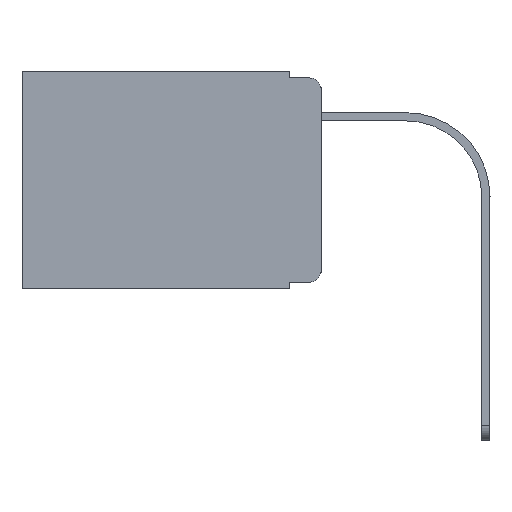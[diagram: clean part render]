
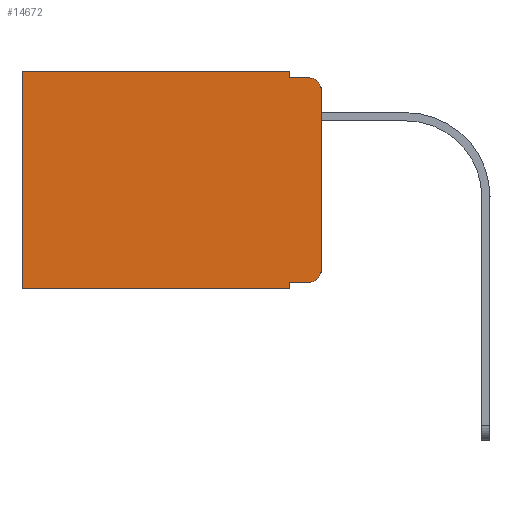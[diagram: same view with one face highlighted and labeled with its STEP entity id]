
A CAD part, left-side view. The second image highlights one B-rep face of the part: STEP entity #14672.
In plain terms, the highlighted planar face has unit normal (-1, 0, 0).
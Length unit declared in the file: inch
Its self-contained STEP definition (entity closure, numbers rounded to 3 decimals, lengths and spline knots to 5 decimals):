
#27 = VERTEX_POINT ( 'NONE', #1675 ) ;
#57 = CARTESIAN_POINT ( 'NONE',  ( 0.298, 0.02, -0.03 ) ) ;
#279 = CARTESIAN_POINT ( 'NONE',  ( 0.298, 0.051, 0. ) ) ;
#735 = ORIENTED_EDGE ( 'NONE', *, *, #15485, .T. ) ;
#769 = VERTEX_POINT ( 'NONE', #1514 ) ;
#1252 = VERTEX_POINT ( 'NONE', #11580 ) ;
#1514 = CARTESIAN_POINT ( 'NONE',  ( 0.298, 0.051, -0.01 ) ) ;
#1627 = PLANE ( 'NONE',  #4900 ) ;
#1675 = CARTESIAN_POINT ( 'NONE',  ( 0.298, 0.051, 0. ) ) ;
#1926 = ORIENTED_EDGE ( 'NONE', *, *, #7723, .T. ) ;
#2039 = EDGE_CURVE ( 'NONE', #3772, #8270, #19873, .T. ) ;
#2563 = VERTEX_POINT ( 'NONE', #8257 ) ;
#2780 = CARTESIAN_POINT ( 'NONE',  ( 0.298, 0.02, -0.01 ) ) ;
#3042 = CIRCLE ( 'NONE', #18244, 0.02 ) ;
#3081 = DIRECTION ( 'NONE',  ( 0., 0., -1. ) ) ;
#3502 = DIRECTION ( 'NONE',  ( 0., 0., -1. ) ) ;
#3566 = LINE ( 'NONE', #17082, #7399 ) ;
#3606 = ORIENTED_EDGE ( 'NONE', *, *, #2039, .T. ) ;
#3688 = LINE ( 'NONE', #20299, #4936 ) ;
#3772 = VERTEX_POINT ( 'NONE', #16902 ) ;
#3963 = LINE ( 'NONE', #7512, #16135 ) ;
#4053 = LINE ( 'NONE', #7702, #10940 ) ;
#4299 = CARTESIAN_POINT ( 'NONE',  ( 0.298, 0.473, 0. ) ) ;
#4418 = DIRECTION ( 'NONE',  ( 0., 0., -1. ) ) ;
#4834 = CARTESIAN_POINT ( 'NONE',  ( 0.298, 0.051, -0.01 ) ) ;
#4900 = AXIS2_PLACEMENT_3D ( 'NONE', #15141, #15360, #3081 ) ;
#4936 = VECTOR ( 'NONE', #20626, 39.37008 ) ;
#5327 = ORIENTED_EDGE ( 'NONE', *, *, #12393, .F. ) ;
#5616 = VECTOR ( 'NONE', #6398, 39.37008 ) ;
#6398 = DIRECTION ( 'NONE',  ( 0., -1., 0. ) ) ;
#6643 = ORIENTED_EDGE ( 'NONE', *, *, #14414, .F. ) ;
#7184 = VERTEX_POINT ( 'NONE', #17137 ) ;
#7365 = EDGE_CURVE ( 'NONE', #27, #10118, #3963, .T. ) ;
#7399 = VECTOR ( 'NONE', #19055, 39.37008 ) ;
#7512 = CARTESIAN_POINT ( 'NONE',  ( 0.298, 0., 0. ) ) ;
#7702 = CARTESIAN_POINT ( 'NONE',  ( 0.298, 0., 0. ) ) ;
#7723 = EDGE_CURVE ( 'NONE', #1252, #19000, #3042, .T. ) ;
#8257 = CARTESIAN_POINT ( 'NONE',  ( 0.298, 0.051, -0.333 ) ) ;
#8270 = VERTEX_POINT ( 'NONE', #9193 ) ;
#8373 = CARTESIAN_POINT ( 'NONE',  ( 0.298, 0.473, 0. ) ) ;
#9161 = DIRECTION ( 'NONE',  ( 0., 1., 0. ) ) ;
#9193 = CARTESIAN_POINT ( 'NONE',  ( 0.298, 0., -0.313 ) ) ;
#9301 = ORIENTED_EDGE ( 'NONE', *, *, #10661, .F. ) ;
#9907 = EDGE_CURVE ( 'NONE', #2563, #3772, #12373, .T. ) ;
#10118 = VERTEX_POINT ( 'NONE', #8373 ) ;
#10119 = EDGE_CURVE ( 'NONE', #769, #19000, #19993, .T. ) ;
#10338 = AXIS2_PLACEMENT_3D ( 'NONE', #13040, #18247, #4418 ) ;
#10351 = EDGE_CURVE ( 'NONE', #1252, #8270, #4053, .T. ) ;
#10617 = CARTESIAN_POINT ( 'NONE',  ( 0.298, 0.051, -0.333 ) ) ;
#10661 = EDGE_CURVE ( 'NONE', #18997, #7184, #3688, .T. ) ;
#10940 = VECTOR ( 'NONE', #16014, 39.37008 ) ;
#11580 = CARTESIAN_POINT ( 'NONE',  ( 0.298, 0., -0.03 ) ) ;
#12355 = VECTOR ( 'NONE', #3502, 39.37008 ) ;
#12373 = LINE ( 'NONE', #10617, #17623 ) ;
#12393 = EDGE_CURVE ( 'NONE', #27, #769, #15458, .T. ) ;
#13040 = CARTESIAN_POINT ( 'NONE',  ( 0.298, 0.02, -0.313 ) ) ;
#13249 = FACE_OUTER_BOUND ( 'NONE', #14753, .T. ) ;
#13452 = DIRECTION ( 'NONE',  ( -1., 0., 0. ) ) ;
#13640 = ORIENTED_EDGE ( 'NONE', *, *, #10119, .F. ) ;
#13667 = DIRECTION ( 'NONE',  ( 0., 0., -1. ) ) ;
#14414 = EDGE_CURVE ( 'NONE', #2563, #18997, #3566, .T. ) ;
#14672 = ADVANCED_FACE ( 'NONE', ( #13249 ), #1627, .F. ) ;
#14753 = EDGE_LOOP ( 'NONE', ( #19637, #1926, #13640, #5327, #19267, #735, #9301, #6643, #16917, #3606 ) ) ;
#14939 = VECTOR ( 'NONE', #19568, 39.37008 ) ;
#15141 = CARTESIAN_POINT ( 'NONE',  ( 0.298, 0., 0. ) ) ;
#15360 = DIRECTION ( 'NONE',  ( 1., 0., 0. ) ) ;
#15458 = LINE ( 'NONE', #279, #12355 ) ;
#15485 = EDGE_CURVE ( 'NONE', #10118, #7184, #16141, .T. ) ;
#16014 = DIRECTION ( 'NONE',  ( 0., 0., -1. ) ) ;
#16135 = VECTOR ( 'NONE', #9161, 39.37008 ) ;
#16141 = LINE ( 'NONE', #4299, #14939 ) ;
#16902 = CARTESIAN_POINT ( 'NONE',  ( 0.298, 0.02, -0.333 ) ) ;
#16917 = ORIENTED_EDGE ( 'NONE', *, *, #9907, .T. ) ;
#17082 = CARTESIAN_POINT ( 'NONE',  ( 0.298, 0.051, 0. ) ) ;
#17137 = CARTESIAN_POINT ( 'NONE',  ( 0.298, 0.473, -0.343 ) ) ;
#17360 = DIRECTION ( 'NONE',  ( 0., -1., 0. ) ) ;
#17623 = VECTOR ( 'NONE', #17360, 39.37008 ) ;
#18244 = AXIS2_PLACEMENT_3D ( 'NONE', #57, #13452, #13667 ) ;
#18247 = DIRECTION ( 'NONE',  ( -1., 0., 0. ) ) ;
#18997 = VERTEX_POINT ( 'NONE', #21381 ) ;
#19000 = VERTEX_POINT ( 'NONE', #2780 ) ;
#19055 = DIRECTION ( 'NONE',  ( 0., 0., -1. ) ) ;
#19267 = ORIENTED_EDGE ( 'NONE', *, *, #7365, .T. ) ;
#19568 = DIRECTION ( 'NONE',  ( 0., 0., -1. ) ) ;
#19637 = ORIENTED_EDGE ( 'NONE', *, *, #10351, .F. ) ;
#19873 = CIRCLE ( 'NONE', #10338, 0.02 ) ;
#19993 = LINE ( 'NONE', #4834, #5616 ) ;
#20299 = CARTESIAN_POINT ( 'NONE',  ( 0.298, 0., -0.343 ) ) ;
#20626 = DIRECTION ( 'NONE',  ( 0., 1., 0. ) ) ;
#21381 = CARTESIAN_POINT ( 'NONE',  ( 0.298, 0.051, -0.343 ) ) ;
